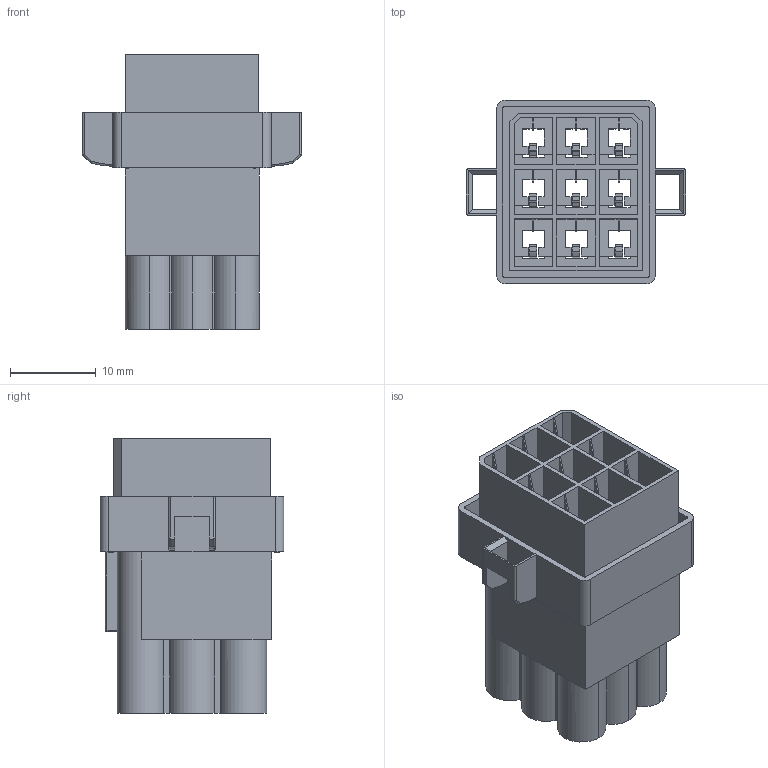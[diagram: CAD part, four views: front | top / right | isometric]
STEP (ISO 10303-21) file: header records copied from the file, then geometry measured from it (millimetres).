
FILE_DESCRIPTION (( 'STEP AP214' ), '1' );
FILE_NAME ('567-009-000-310.STEP', '2020-07-27T20:20:15', ( '' ), ( '' ), 'SwSTEP 2.0', 'SolidWorks 2020', '' );
FILE_SCHEMA (( 'AUTOMOTIVE_DESIGN' ));
Length unit declared in the file: millimetre
Products named in the file (1): 567-009-000-310
Bounding box: 25.5 x 21.4 x 32 mm (x, y, z)
Volume: 3767.6 mm3; surface area: 9814.8 mm2
Topology: 1 solids, 13 shells, 688 faces, 1903 edges, 1250 vertices
Faces by surface type: plane 571, cylinder 82, bspline 29, torus 4, sphere 2
Entity records: 23245 total; most frequent: CARTESIAN_POINT 5706, ORIENTED_EDGE 3802, DIRECTION 3359, EDGE_CURVE 1901, LINE 1577, VECTOR 1577, VERTEX_POINT 1250, AXIS2_PLACEMENT_3D 891
